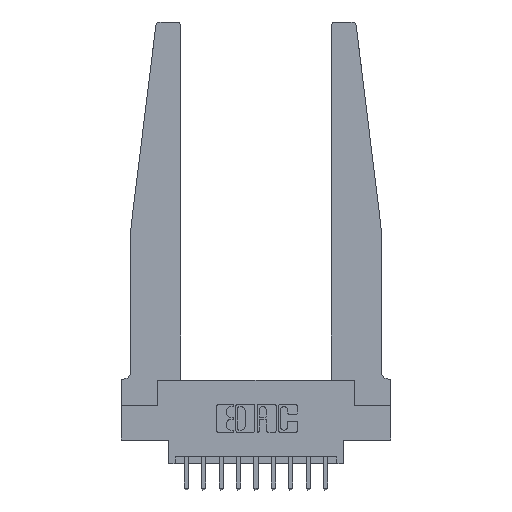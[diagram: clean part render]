
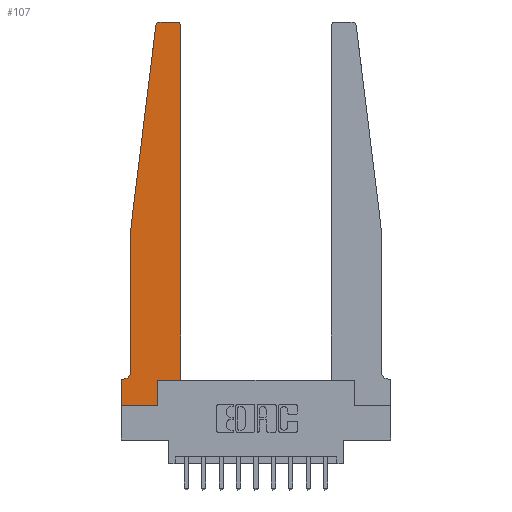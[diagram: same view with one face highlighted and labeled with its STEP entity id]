
A CAD part, top view. The second image highlights one B-rep face of the part: STEP entity #107.
In plain terms, the highlighted planar face has unit normal (0, 0, 1).
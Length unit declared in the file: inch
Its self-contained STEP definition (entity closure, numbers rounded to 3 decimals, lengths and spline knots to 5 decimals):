
#94 = DIRECTION ( 'NONE',  ( 0., -1., 0. ) ) ;
#107 = ADVANCED_FACE ( 'NONE', ( #3414 ), #3950, .T. ) ;
#109 = ORIENTED_EDGE ( 'NONE', *, *, #4000, .T. ) ;
#124 = VECTOR ( 'NONE', #10000, 39.37008 ) ;
#260 = ORIENTED_EDGE ( 'NONE', *, *, #14601, .T. ) ;
#625 = ORIENTED_EDGE ( 'NONE', *, *, #3190, .T. ) ;
#884 = VERTEX_POINT ( 'NONE', #10364 ) ;
#947 = EDGE_CURVE ( 'NONE', #8875, #10041, #14668, .T. ) ;
#996 = AXIS2_PLACEMENT_3D ( 'NONE', #5928, #10218, #9341 ) ;
#1282 = CARTESIAN_POINT ( 'NONE',  ( 0.065, 0.2375, 0.37 ) ) ;
#1335 = VERTEX_POINT ( 'NONE', #14326 ) ;
#1426 = AXIS2_PLACEMENT_3D ( 'NONE', #1593, #9850, #2790 ) ;
#1593 = CARTESIAN_POINT ( 'NONE',  ( 0.395, 2.72, 0.37 ) ) ;
#1670 = VERTEX_POINT ( 'NONE', #9999 ) ;
#1703 = EDGE_CURVE ( 'NONE', #5351, #15224, #14844, .T. ) ;
#1848 = VECTOR ( 'NONE', #10226, 39.37008 ) ;
#1914 = EDGE_CURVE ( 'NONE', #1335, #4212, #9457, .T. ) ;
#1997 = ORIENTED_EDGE ( 'NONE', *, *, #14479, .T. ) ;
#2198 = DIRECTION ( 'NONE',  ( -0.122, -0.992, 0. ) ) ;
#2222 = LINE ( 'NONE', #12499, #1848 ) ;
#2229 = VECTOR ( 'NONE', #2606, 39.37008 ) ;
#2606 = DIRECTION ( 'NONE',  ( 1., 0., 0. ) ) ;
#2790 = DIRECTION ( 'NONE',  ( 1., 0., 0. ) ) ;
#3146 = CARTESIAN_POINT ( 'NONE',  ( 0.27653, 2.75, 0.37 ) ) ;
#3189 = VECTOR ( 'NONE', #7422, 39.37008 ) ;
#3190 = EDGE_CURVE ( 'NONE', #884, #1335, #5947, .T. ) ;
#3414 = FACE_OUTER_BOUND ( 'NONE', #5283, .T. ) ;
#3731 = CARTESIAN_POINT ( 'NONE',  ( 0.015, 0.2375, 0.37 ) ) ;
#3758 = CARTESIAN_POINT ( 'NONE',  ( 0.425, 0.18, 0.37 ) ) ;
#3950 = PLANE ( 'NONE',  #996 ) ;
#4000 = EDGE_CURVE ( 'NONE', #10041, #8800, #2222, .T. ) ;
#4154 = CARTESIAN_POINT ( 'NONE',  ( 0.2605, 0.18, 0.37 ) ) ;
#4212 = VERTEX_POINT ( 'NONE', #8251 ) ;
#4314 = VERTEX_POINT ( 'NONE', #1282 ) ;
#4790 = CARTESIAN_POINT ( 'NONE',  ( 0.27653, 2.72, 0.37 ) ) ;
#4846 = CARTESIAN_POINT ( 'NONE',  ( 0.395, 2.75, 0.37 ) ) ;
#4924 = DIRECTION ( 'NONE',  ( -1., 0., 0. ) ) ;
#5283 = EDGE_LOOP ( 'NONE', ( #11797, #5746, #12531, #11603, #1997, #11050, #109, #7028, #7576, #625, #11350, #260 ) ) ;
#5351 = VERTEX_POINT ( 'NONE', #4846 ) ;
#5420 = VECTOR ( 'NONE', #9471, 39.37008 ) ;
#5564 = VECTOR ( 'NONE', #94, 39.37008 ) ;
#5586 = VECTOR ( 'NONE', #13189, 39.37008 ) ;
#5724 = EDGE_CURVE ( 'NONE', #1670, #12525, #14546, .T. ) ;
#5746 = ORIENTED_EDGE ( 'NONE', *, *, #13772, .T. ) ;
#5928 = CARTESIAN_POINT ( 'NONE',  ( 0., 0.1875, 0.37 ) ) ;
#5947 = LINE ( 'NONE', #3758, #5586 ) ;
#5971 = DIRECTION ( 'NONE',  ( 1., 0., 0. ) ) ;
#6686 = CIRCLE ( 'NONE', #8854, 0.05 ) ;
#6782 = CARTESIAN_POINT ( 'NONE',  ( 0., 0.1875, 0.37 ) ) ;
#7028 = ORIENTED_EDGE ( 'NONE', *, *, #9127, .T. ) ;
#7422 = DIRECTION ( 'NONE',  ( 0., 1., 0. ) ) ;
#7518 = CARTESIAN_POINT ( 'NONE',  ( 0.425, 0.18, 0.37 ) ) ;
#7576 = ORIENTED_EDGE ( 'NONE', *, *, #9895, .T. ) ;
#8251 = CARTESIAN_POINT ( 'NONE',  ( 0.425, 2.72, 0.37 ) ) ;
#8292 = VECTOR ( 'NONE', #2198, 39.37008 ) ;
#8357 = CIRCLE ( 'NONE', #1426, 0.03 ) ;
#8662 = AXIS2_PLACEMENT_3D ( 'NONE', #4790, #13025, #5971 ) ;
#8696 = LINE ( 'NONE', #11890, #5564 ) ;
#8706 = DIRECTION ( 'NONE',  ( -1., 0., 0. ) ) ;
#8800 = VERTEX_POINT ( 'NONE', #14974 ) ;
#8854 = AXIS2_PLACEMENT_3D ( 'NONE', #3731, #11958, #4924 ) ;
#8875 = VERTEX_POINT ( 'NONE', #13923 ) ;
#9015 = CARTESIAN_POINT ( 'NONE',  ( 0.065, 0.1875, 0.37 ) ) ;
#9127 = EDGE_CURVE ( 'NONE', #8800, #15180, #12935, .T. ) ;
#9238 = CARTESIAN_POINT ( 'NONE',  ( 0.065, 1.25, 0.37 ) ) ;
#9341 = DIRECTION ( 'NONE',  ( 1., 0., 0. ) ) ;
#9457 = LINE ( 'NONE', #7518, #3189 ) ;
#9458 = CARTESIAN_POINT ( 'NONE',  ( 0.25, 2.75, 0.37 ) ) ;
#9471 = DIRECTION ( 'NONE',  ( -1., 0., 0. ) ) ;
#9665 = CARTESIAN_POINT ( 'NONE',  ( 0., 0., 0.37 ) ) ;
#9850 = DIRECTION ( 'NONE',  ( 0., 0., 1. ) ) ;
#9895 = EDGE_CURVE ( 'NONE', #15180, #884, #13096, .T. ) ;
#9926 = CARTESIAN_POINT ( 'NONE',  ( 0.2605, 0., 0.37 ) ) ;
#9999 = CARTESIAN_POINT ( 'NONE',  ( 0.24675, 2.72367, 0.37 ) ) ;
#10000 = DIRECTION ( 'NONE',  ( 0., 1., 0. ) ) ;
#10041 = VERTEX_POINT ( 'NONE', #6782 ) ;
#10218 = DIRECTION ( 'NONE',  ( 0., 0., 1. ) ) ;
#10226 = DIRECTION ( 'NONE',  ( 0., -1., 0. ) ) ;
#10364 = CARTESIAN_POINT ( 'NONE',  ( 0.2605, 0.18, 0.37 ) ) ;
#11050 = ORIENTED_EDGE ( 'NONE', *, *, #947, .T. ) ;
#11350 = ORIENTED_EDGE ( 'NONE', *, *, #1914, .T. ) ;
#11501 = VECTOR ( 'NONE', #8706, 39.37008 ) ;
#11603 = ORIENTED_EDGE ( 'NONE', *, *, #14990, .T. ) ;
#11797 = ORIENTED_EDGE ( 'NONE', *, *, #1703, .T. ) ;
#11890 = CARTESIAN_POINT ( 'NONE',  ( 0.065, 1.25, 0.37 ) ) ;
#11958 = DIRECTION ( 'NONE',  ( 0., 0., -1. ) ) ;
#12404 = CIRCLE ( 'NONE', #8662, 0.03 ) ;
#12499 = CARTESIAN_POINT ( 'NONE',  ( 0., 0., 0.37 ) ) ;
#12525 = VERTEX_POINT ( 'NONE', #9238 ) ;
#12531 = ORIENTED_EDGE ( 'NONE', *, *, #5724, .T. ) ;
#12935 = LINE ( 'NONE', #9665, #2229 ) ;
#13025 = DIRECTION ( 'NONE',  ( 0., 0., 1. ) ) ;
#13096 = LINE ( 'NONE', #4154, #124 ) ;
#13189 = DIRECTION ( 'NONE',  ( 1., 0., 0. ) ) ;
#13772 = EDGE_CURVE ( 'NONE', #15224, #1670, #12404, .T. ) ;
#13923 = CARTESIAN_POINT ( 'NONE',  ( 0.015, 0.1875, 0.37 ) ) ;
#14326 = CARTESIAN_POINT ( 'NONE',  ( 0.425, 0.18, 0.37 ) ) ;
#14479 = EDGE_CURVE ( 'NONE', #4314, #8875, #6686, .T. ) ;
#14546 = LINE ( 'NONE', #15160, #8292 ) ;
#14601 = EDGE_CURVE ( 'NONE', #4212, #5351, #8357, .T. ) ;
#14668 = LINE ( 'NONE', #9015, #11501 ) ;
#14844 = LINE ( 'NONE', #9458, #5420 ) ;
#14974 = CARTESIAN_POINT ( 'NONE',  ( 0., 0., 0.37 ) ) ;
#14990 = EDGE_CURVE ( 'NONE', #12525, #4314, #8696, .T. ) ;
#15160 = CARTESIAN_POINT ( 'NONE',  ( 0.065, 1.25, 0.37 ) ) ;
#15180 = VERTEX_POINT ( 'NONE', #9926 ) ;
#15224 = VERTEX_POINT ( 'NONE', #3146 ) ;
